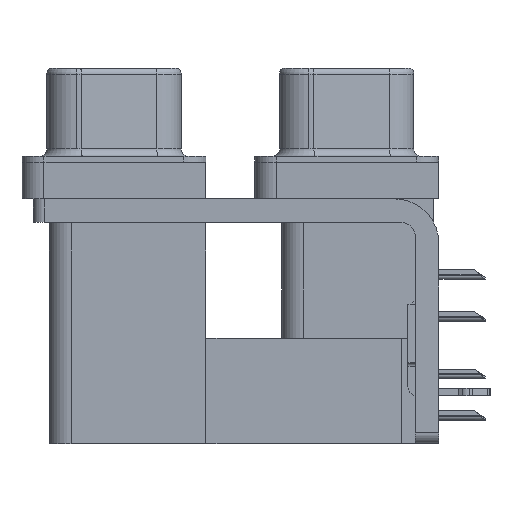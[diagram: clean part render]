
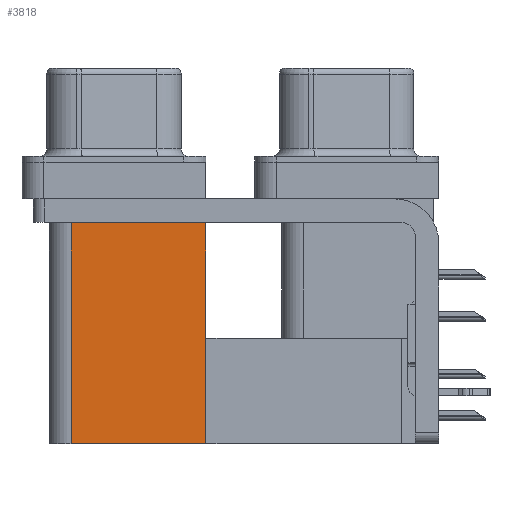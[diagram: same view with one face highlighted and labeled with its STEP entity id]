
A CAD part, left-side view. The second image highlights one B-rep face of the part: STEP entity #3818.
In plain terms, the highlighted planar face has unit normal (-1, 0, 0).
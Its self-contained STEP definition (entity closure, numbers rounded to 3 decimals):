
#2008 = VECTOR ( 'NONE', #26153, 1000. ) ;
#3507 = ORIENTED_EDGE ( 'NONE', *, *, #43885, .T. ) ;
#3633 = PLANE ( 'NONE',  #28511 ) ;
#3818 = ADVANCED_FACE ( 'NONE', ( #33925 ), #3633, .F. ) ;
#5311 = ORIENTED_EDGE ( 'NONE', *, *, #15543, .F. ) ;
#7467 = LINE ( 'NONE', #46160, #43051 ) ;
#7545 = CARTESIAN_POINT ( 'NONE',  ( 3.79, 18.8, -2.5 ) ) ;
#9216 = VERTEX_POINT ( 'NONE', #33854 ) ;
#9638 = EDGE_CURVE ( 'NONE', #9216, #44710, #38106, .T. ) ;
#14089 = ORIENTED_EDGE ( 'NONE', *, *, #9638, .T. ) ;
#14594 = DIRECTION ( 'NONE',  ( 0., 1., 0. ) ) ;
#15106 = LINE ( 'NONE', #41558, #42244 ) ;
#15543 = EDGE_CURVE ( 'NONE', #26632, #44990, #7467, .T. ) ;
#15868 = DIRECTION ( 'NONE',  ( 0., 0., 1. ) ) ;
#16431 = CARTESIAN_POINT ( 'NONE',  ( 3.79, 9.6, -2.5 ) ) ;
#18652 = DIRECTION ( 'NONE',  ( 0., 0., -1. ) ) ;
#18718 = EDGE_LOOP ( 'NONE', ( #3507, #5311, #41937, #14089 ) ) ;
#22715 = CARTESIAN_POINT ( 'NONE',  ( 3.79, 9.6, -19.2 ) ) ;
#26153 = DIRECTION ( 'NONE',  ( 0., 0., 1. ) ) ;
#26632 = VERTEX_POINT ( 'NONE', #43688 ) ;
#28467 = CARTESIAN_POINT ( 'NONE',  ( 3.79, 9.6, -2.5 ) ) ;
#28511 = AXIS2_PLACEMENT_3D ( 'NONE', #22715, #38238, #18652 ) ;
#33047 = CARTESIAN_POINT ( 'NONE',  ( 3.79, 9.6, -19.2 ) ) ;
#33854 = CARTESIAN_POINT ( 'NONE',  ( 3.79, 9.6, -19.2 ) ) ;
#33925 = FACE_OUTER_BOUND ( 'NONE', #18718, .T. ) ;
#36280 = LINE ( 'NONE', #16431, #39484 ) ;
#38106 = LINE ( 'NONE', #33047, #2008 ) ;
#38238 = DIRECTION ( 'NONE',  ( 1., 0., 0. ) ) ;
#39484 = VECTOR ( 'NONE', #44402, 1000. ) ;
#39818 = EDGE_CURVE ( 'NONE', #9216, #26632, #15106, .T. ) ;
#41558 = CARTESIAN_POINT ( 'NONE',  ( 3.79, 9.6, -19.2 ) ) ;
#41937 = ORIENTED_EDGE ( 'NONE', *, *, #39818, .F. ) ;
#42244 = VECTOR ( 'NONE', #14594, 1000. ) ;
#43051 = VECTOR ( 'NONE', #15868, 1000. ) ;
#43688 = CARTESIAN_POINT ( 'NONE',  ( 3.79, 18.8, -19.2 ) ) ;
#43885 = EDGE_CURVE ( 'NONE', #44710, #44990, #36280, .T. ) ;
#44402 = DIRECTION ( 'NONE',  ( 0., 1., 0. ) ) ;
#44710 = VERTEX_POINT ( 'NONE', #28467 ) ;
#44990 = VERTEX_POINT ( 'NONE', #7545 ) ;
#46160 = CARTESIAN_POINT ( 'NONE',  ( 3.79, 18.8, -19.2 ) ) ;
